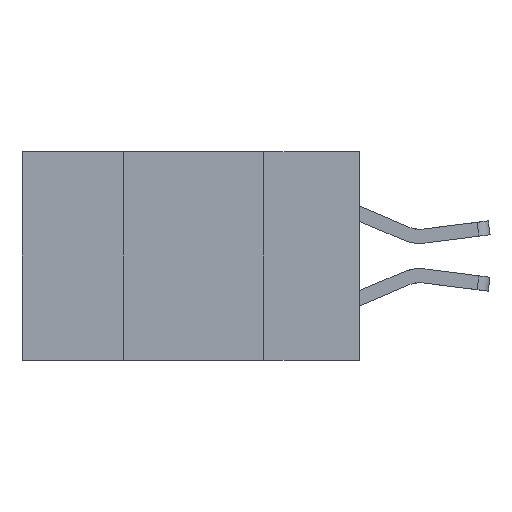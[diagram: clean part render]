
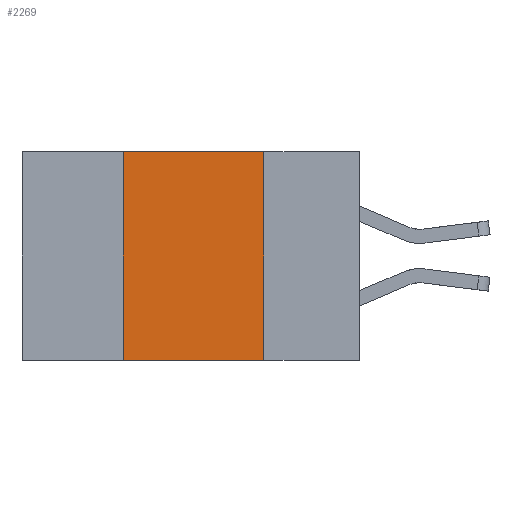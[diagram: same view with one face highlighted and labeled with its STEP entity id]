
A CAD part, left-side view. The second image highlights one B-rep face of the part: STEP entity #2269.
In plain terms, the highlighted planar face has unit normal (-1, 0, 0).
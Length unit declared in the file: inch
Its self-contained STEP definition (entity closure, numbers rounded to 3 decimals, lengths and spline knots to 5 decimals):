
#27 = VECTOR ( 'NONE', #8944, 39.37008 ) ;
#1079 = EDGE_CURVE ( 'NONE', #3976, #10013, #3042, .T. ) ;
#1360 = EDGE_CURVE ( 'NONE', #8387, #6744, #5175, .T. ) ;
#1559 = CARTESIAN_POINT ( 'NONE',  ( 0., 0.42, 0. ) ) ;
#1634 = CARTESIAN_POINT ( 'NONE',  ( 0., 0.17, 0. ) ) ;
#1717 = FACE_OUTER_BOUND ( 'NONE', #6138, .T. ) ;
#1738 = DIRECTION ( 'NONE',  ( 0., -1., 0. ) ) ;
#1935 = CARTESIAN_POINT ( 'NONE',  ( 0., 0.17, 0. ) ) ;
#2105 = ORIENTED_EDGE ( 'NONE', *, *, #2964, .F. ) ;
#2269 = ADVANCED_FACE ( 'NONE', ( #1717 ), #7814, .F. ) ;
#2439 = EDGE_CURVE ( 'NONE', #10013, #6744, #5599, .T. ) ;
#2788 = VECTOR ( 'NONE', #6433, 39.37008 ) ;
#2800 = VECTOR ( 'NONE', #2840, 39.37008 ) ;
#2840 = DIRECTION ( 'NONE',  ( 0., 0., 1. ) ) ;
#2964 = EDGE_CURVE ( 'NONE', #8387, #3976, #7081, .T. ) ;
#3042 = LINE ( 'NONE', #9824, #27 ) ;
#3976 = VERTEX_POINT ( 'NONE', #1559 ) ;
#4393 = AXIS2_PLACEMENT_3D ( 'NONE', #4463, #5152, #6848 ) ;
#4463 = CARTESIAN_POINT ( 'NONE',  ( 0., 0.6, 0. ) ) ;
#4782 = ORIENTED_EDGE ( 'NONE', *, *, #1360, .T. ) ;
#4896 = CARTESIAN_POINT ( 'NONE',  ( 0., 0.42, -0.37 ) ) ;
#5152 = DIRECTION ( 'NONE',  ( 1., 0., 0. ) ) ;
#5175 = LINE ( 'NONE', #5229, #9169 ) ;
#5229 = CARTESIAN_POINT ( 'NONE',  ( 0., 0.6, -0.37 ) ) ;
#5599 = LINE ( 'NONE', #1935, #2788 ) ;
#6138 = EDGE_LOOP ( 'NONE', ( #8751, #9241, #2105, #4782 ) ) ;
#6433 = DIRECTION ( 'NONE',  ( 0., 0., -1. ) ) ;
#6744 = VERTEX_POINT ( 'NONE', #9649 ) ;
#6848 = DIRECTION ( 'NONE',  ( 0., 0., -1. ) ) ;
#7081 = LINE ( 'NONE', #9575, #2800 ) ;
#7814 = PLANE ( 'NONE',  #4393 ) ;
#8387 = VERTEX_POINT ( 'NONE', #4896 ) ;
#8751 = ORIENTED_EDGE ( 'NONE', *, *, #2439, .F. ) ;
#8944 = DIRECTION ( 'NONE',  ( 0., -1., 0. ) ) ;
#9169 = VECTOR ( 'NONE', #1738, 39.37008 ) ;
#9241 = ORIENTED_EDGE ( 'NONE', *, *, #1079, .F. ) ;
#9575 = CARTESIAN_POINT ( 'NONE',  ( 0., 0.42, 0. ) ) ;
#9649 = CARTESIAN_POINT ( 'NONE',  ( 0., 0.17, -0.37 ) ) ;
#9824 = CARTESIAN_POINT ( 'NONE',  ( 0., 0.6, 0. ) ) ;
#10013 = VERTEX_POINT ( 'NONE', #1634 ) ;
